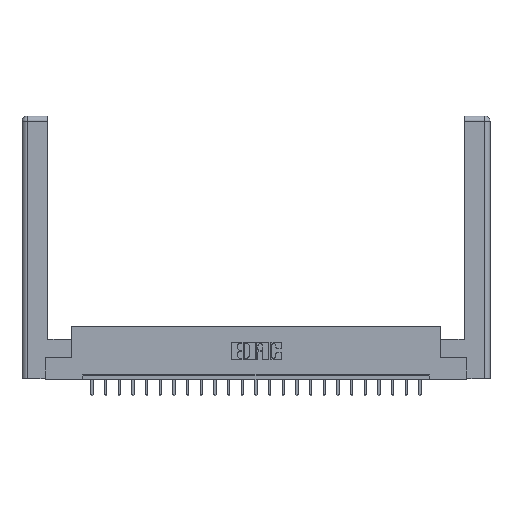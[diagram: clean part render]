
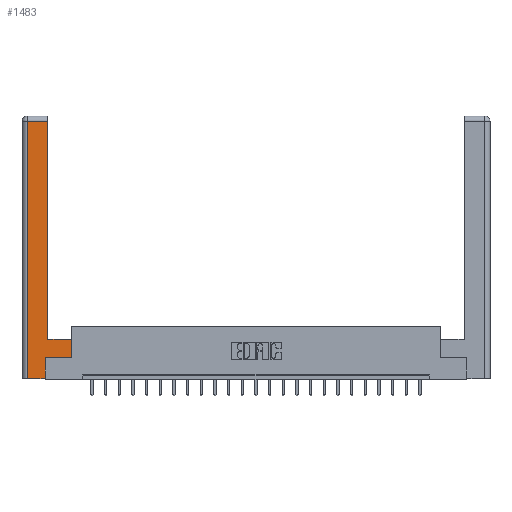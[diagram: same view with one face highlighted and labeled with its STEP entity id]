
A CAD part, top view. The second image highlights one B-rep face of the part: STEP entity #1483.
In plain terms, the highlighted planar face has unit normal (0, 0, 1).
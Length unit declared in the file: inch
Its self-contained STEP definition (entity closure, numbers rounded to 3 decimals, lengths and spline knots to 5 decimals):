
#420 = DIRECTION ( 'NONE',  ( 0., 1., 0. ) ) ;
#641 = DIRECTION ( 'NONE',  ( -1., 0., 0. ) ) ;
#870 = ORIENTED_EDGE ( 'NONE', *, *, #16227, .T. ) ;
#1302 = EDGE_CURVE ( 'NONE', #8900, #14586, #16608, .T. ) ;
#1483 = ADVANCED_FACE ( 'NONE', ( #22040 ), #15464, .F. ) ;
#2091 = CARTESIAN_POINT ( 'NONE',  ( 0.295, 2.94, 0. ) ) ;
#2604 = DIRECTION ( 'NONE',  ( 0., 0., -1. ) ) ;
#2810 = VECTOR ( 'NONE', #11600, 39.37008 ) ;
#2823 = EDGE_LOOP ( 'NONE', ( #14192, #22853, #870, #9349, #8748, #14330, #10132, #10780 ) ) ;
#3308 = EDGE_CURVE ( 'NONE', #10522, #20248, #20569, .T. ) ;
#3950 = DIRECTION ( 'NONE',  ( 1., 0., 0. ) ) ;
#4084 = VECTOR ( 'NONE', #17956, 39.37008 ) ;
#4397 = VECTOR ( 'NONE', #3950, 39.37008 ) ;
#4684 = DIRECTION ( 'NONE',  ( -1., 0., 0. ) ) ;
#5033 = VECTOR ( 'NONE', #21807, 39.37008 ) ;
#5410 = CARTESIAN_POINT ( 'NONE',  ( 0.565, 0.245, 0. ) ) ;
#5423 = CARTESIAN_POINT ( 'NONE',  ( 0.565, 0.45, 0. ) ) ;
#6204 = DIRECTION ( 'NONE',  ( 0., -1., 0. ) ) ;
#6528 = CARTESIAN_POINT ( 'NONE',  ( 0.565, 0.45, 0. ) ) ;
#7021 = LINE ( 'NONE', #11286, #12126 ) ;
#7054 = VERTEX_POINT ( 'NONE', #16362 ) ;
#7451 = VERTEX_POINT ( 'NONE', #9372 ) ;
#8748 = ORIENTED_EDGE ( 'NONE', *, *, #12836, .T. ) ;
#8900 = VERTEX_POINT ( 'NONE', #20717 ) ;
#9203 = VERTEX_POINT ( 'NONE', #23492 ) ;
#9349 = ORIENTED_EDGE ( 'NONE', *, *, #1302, .T. ) ;
#9372 = CARTESIAN_POINT ( 'NONE',  ( 0.295, 0.45, 0. ) ) ;
#9795 = CARTESIAN_POINT ( 'NONE',  ( 0.565, 0.245, 0. ) ) ;
#10132 = ORIENTED_EDGE ( 'NONE', *, *, #3308, .T. ) ;
#10522 = VERTEX_POINT ( 'NONE', #5410 ) ;
#10624 = VERTEX_POINT ( 'NONE', #2091 ) ;
#10780 = ORIENTED_EDGE ( 'NONE', *, *, #16174, .T. ) ;
#10827 = EDGE_CURVE ( 'NONE', #9203, #10522, #15041, .T. ) ;
#11286 = CARTESIAN_POINT ( 'NONE',  ( 0.265, 0.245, 0. ) ) ;
#11504 = CARTESIAN_POINT ( 'NONE',  ( 0., 0., 0. ) ) ;
#11600 = DIRECTION ( 'NONE',  ( 1., 0., 0. ) ) ;
#12126 = VECTOR ( 'NONE', #420, 39.37008 ) ;
#12617 = CARTESIAN_POINT ( 'NONE',  ( 0.0615, 2.94, 0. ) ) ;
#12695 = EDGE_CURVE ( 'NONE', #10624, #7054, #13292, .T. ) ;
#12836 = EDGE_CURVE ( 'NONE', #14586, #9203, #7021, .T. ) ;
#13251 = LINE ( 'NONE', #21256, #13824 ) ;
#13292 = LINE ( 'NONE', #12617, #5033 ) ;
#13339 = EDGE_CURVE ( 'NONE', #7451, #10624, #13251, .T. ) ;
#13672 = CARTESIAN_POINT ( 'NONE',  ( 0.265, 0., 0. ) ) ;
#13751 = CARTESIAN_POINT ( 'NONE',  ( 0.0615, 0., 0. ) ) ;
#13824 = VECTOR ( 'NONE', #14253, 39.37008 ) ;
#14192 = ORIENTED_EDGE ( 'NONE', *, *, #13339, .T. ) ;
#14253 = DIRECTION ( 'NONE',  ( 0., 1., 0. ) ) ;
#14330 = ORIENTED_EDGE ( 'NONE', *, *, #10827, .T. ) ;
#14586 = VERTEX_POINT ( 'NONE', #13672 ) ;
#14592 = VECTOR ( 'NONE', #4684, 39.37008 ) ;
#15041 = LINE ( 'NONE', #9795, #2810 ) ;
#15461 = LINE ( 'NONE', #13751, #19144 ) ;
#15464 = PLANE ( 'NONE',  #17081 ) ;
#16174 = EDGE_CURVE ( 'NONE', #20248, #7451, #20576, .T. ) ;
#16227 = EDGE_CURVE ( 'NONE', #7054, #8900, #15461, .T. ) ;
#16362 = CARTESIAN_POINT ( 'NONE',  ( 0.0615, 2.94, 0. ) ) ;
#16608 = LINE ( 'NONE', #20327, #4397 ) ;
#17081 = AXIS2_PLACEMENT_3D ( 'NONE', #11504, #2604, #641 ) ;
#17956 = DIRECTION ( 'NONE',  ( 0., 1., 0. ) ) ;
#19144 = VECTOR ( 'NONE', #6204, 39.37008 ) ;
#20248 = VERTEX_POINT ( 'NONE', #6528 ) ;
#20327 = CARTESIAN_POINT ( 'NONE',  ( 0.265, 0., 0. ) ) ;
#20569 = LINE ( 'NONE', #5423, #4084 ) ;
#20576 = LINE ( 'NONE', #22825, #14592 ) ;
#20717 = CARTESIAN_POINT ( 'NONE',  ( 0.0615, 0., 0. ) ) ;
#21256 = CARTESIAN_POINT ( 'NONE',  ( 0.295, 3., 0. ) ) ;
#21807 = DIRECTION ( 'NONE',  ( -1., 0., 0. ) ) ;
#22040 = FACE_OUTER_BOUND ( 'NONE', #2823, .T. ) ;
#22825 = CARTESIAN_POINT ( 'NONE',  ( 0.295, 0.45, 0. ) ) ;
#22853 = ORIENTED_EDGE ( 'NONE', *, *, #12695, .T. ) ;
#23492 = CARTESIAN_POINT ( 'NONE',  ( 0.265, 0.245, 0. ) ) ;
